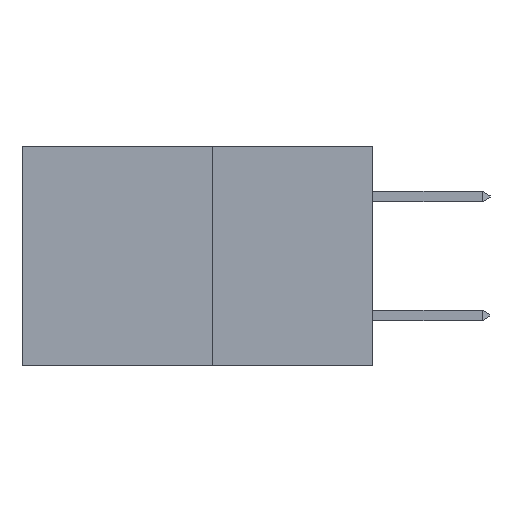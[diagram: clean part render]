
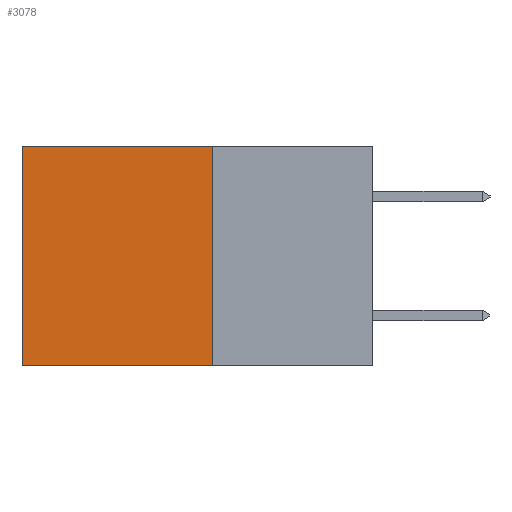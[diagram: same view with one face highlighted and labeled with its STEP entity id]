
A CAD part, left-side view. The second image highlights one B-rep face of the part: STEP entity #3078.
In plain terms, the highlighted planar face has unit normal (-1, 0, 0).
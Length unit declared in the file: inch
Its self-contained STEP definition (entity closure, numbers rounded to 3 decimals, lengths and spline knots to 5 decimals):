
#323 = LINE ( 'NONE', #5892, #2171 ) ;
#431 = EDGE_LOOP ( 'NONE', ( #5180, #3197, #9184, #3427 ) ) ;
#730 = VECTOR ( 'NONE', #7098, 39.37008 ) ;
#878 = CARTESIAN_POINT ( 'NONE',  ( 0.277, 0.27, -0.37 ) ) ;
#1045 = AXIS2_PLACEMENT_3D ( 'NONE', #878, #5797, #5463 ) ;
#1989 = LINE ( 'NONE', #2247, #5896 ) ;
#2171 = VECTOR ( 'NONE', #6720, 39.37008 ) ;
#2247 = CARTESIAN_POINT ( 'NONE',  ( 0.277, 0.27, 0. ) ) ;
#2263 = VERTEX_POINT ( 'NONE', #2453 ) ;
#2453 = CARTESIAN_POINT ( 'NONE',  ( 0.277, 0.27, 0. ) ) ;
#3078 = ADVANCED_FACE ( 'NONE', ( #9017 ), #4080, .F. ) ;
#3197 = ORIENTED_EDGE ( 'NONE', *, *, #3441, .F. ) ;
#3427 = ORIENTED_EDGE ( 'NONE', *, *, #8282, .T. ) ;
#3441 = EDGE_CURVE ( 'NONE', #5311, #9178, #4774, .T. ) ;
#3609 = EDGE_CURVE ( 'NONE', #2263, #5311, #7009, .T. ) ;
#4000 = CARTESIAN_POINT ( 'NONE',  ( 0.277, 0.27, -0.37 ) ) ;
#4080 = PLANE ( 'NONE',  #1045 ) ;
#4610 = VERTEX_POINT ( 'NONE', #6333 ) ;
#4774 = LINE ( 'NONE', #8969, #730 ) ;
#4829 = DIRECTION ( 'NONE',  ( 0., 0., -1. ) ) ;
#4949 = CARTESIAN_POINT ( 'NONE',  ( 0.277, 0.27, -0.37 ) ) ;
#5125 = VECTOR ( 'NONE', #4829, 39.37008 ) ;
#5180 = ORIENTED_EDGE ( 'NONE', *, *, #5521, .T. ) ;
#5311 = VERTEX_POINT ( 'NONE', #4000 ) ;
#5463 = DIRECTION ( 'NONE',  ( 0., 0., -1. ) ) ;
#5521 = EDGE_CURVE ( 'NONE', #4610, #9178, #323, .T. ) ;
#5797 = DIRECTION ( 'NONE',  ( 1., 0., 0. ) ) ;
#5892 = CARTESIAN_POINT ( 'NONE',  ( 0.277, 0.59, -0.37 ) ) ;
#5896 = VECTOR ( 'NONE', #7393, 39.37008 ) ;
#6333 = CARTESIAN_POINT ( 'NONE',  ( 0.277, 0.59, 0. ) ) ;
#6356 = CARTESIAN_POINT ( 'NONE',  ( 0.277, 0.59, -0.37 ) ) ;
#6720 = DIRECTION ( 'NONE',  ( 0., 0., -1. ) ) ;
#7009 = LINE ( 'NONE', #4949, #5125 ) ;
#7098 = DIRECTION ( 'NONE',  ( 0., 1., 0. ) ) ;
#7393 = DIRECTION ( 'NONE',  ( 0., 1., 0. ) ) ;
#8282 = EDGE_CURVE ( 'NONE', #2263, #4610, #1989, .T. ) ;
#8969 = CARTESIAN_POINT ( 'NONE',  ( 0.277, 0.27, -0.37 ) ) ;
#9017 = FACE_OUTER_BOUND ( 'NONE', #431, .T. ) ;
#9178 = VERTEX_POINT ( 'NONE', #6356 ) ;
#9184 = ORIENTED_EDGE ( 'NONE', *, *, #3609, .F. ) ;
